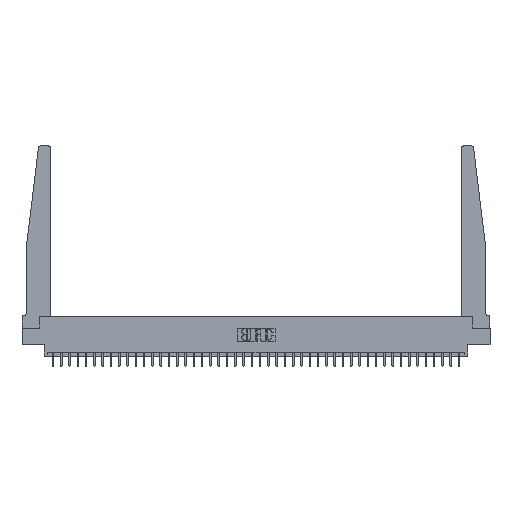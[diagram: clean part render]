
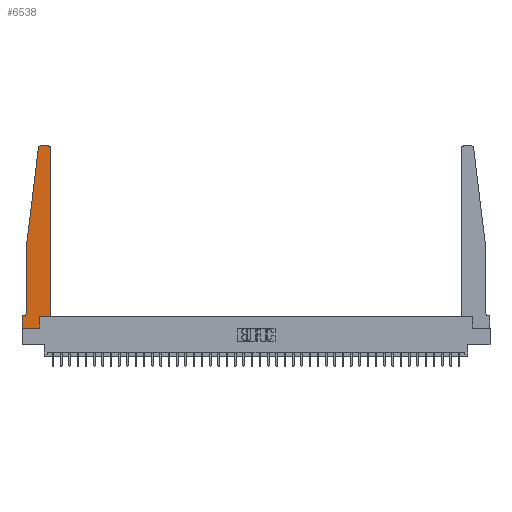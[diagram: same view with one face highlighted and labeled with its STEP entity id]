
A CAD part, top view. The second image highlights one B-rep face of the part: STEP entity #6538.
In plain terms, the highlighted planar face has unit normal (0, 0, 1).
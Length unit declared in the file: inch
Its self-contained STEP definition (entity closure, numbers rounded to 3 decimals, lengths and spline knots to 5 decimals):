
#1526 = CARTESIAN_POINT ( 'NONE',  ( 0.395, 2.72, 0.37 ) ) ;
#1542 = DIRECTION ( 'NONE',  ( 0., 0., -1. ) ) ;
#1617 = LINE ( 'NONE', #13007, #29551 ) ;
#2048 = ORIENTED_EDGE ( 'NONE', *, *, #34001, .T. ) ;
#3100 = EDGE_LOOP ( 'NONE', ( #33316, #14852, #31271, #36779, #28661, #2048, #5179, #14678, #21948, #8942, #9484, #10486 ) ) ;
#3137 = CARTESIAN_POINT ( 'NONE',  ( 0.2605, 0.18, 0.37 ) ) ;
#3719 = VECTOR ( 'NONE', #31763, 39.37008 ) ;
#3794 = VERTEX_POINT ( 'NONE', #31771 ) ;
#3957 = CARTESIAN_POINT ( 'NONE',  ( 0.27653, 2.75, 0.37 ) ) ;
#4169 = EDGE_CURVE ( 'NONE', #3794, #10725, #15048, .T. ) ;
#4283 = PLANE ( 'NONE',  #24182 ) ;
#4781 = DIRECTION ( 'NONE',  ( -1., 0., 0. ) ) ;
#5073 = VECTOR ( 'NONE', #5167, 39.37008 ) ;
#5167 = DIRECTION ( 'NONE',  ( 0., -1., 0. ) ) ;
#5179 = ORIENTED_EDGE ( 'NONE', *, *, #28534, .T. ) ;
#5540 = LINE ( 'NONE', #5727, #5073 ) ;
#5547 = VERTEX_POINT ( 'NONE', #3137 ) ;
#5727 = CARTESIAN_POINT ( 'NONE',  ( 0., 0., 0.37 ) ) ;
#5973 = VECTOR ( 'NONE', #20442, 39.37008 ) ;
#6538 = ADVANCED_FACE ( 'NONE', ( #36244 ), #4283, .T. ) ;
#6959 = DIRECTION ( 'NONE',  ( 0., 0., 1. ) ) ;
#6969 = DIRECTION ( 'NONE',  ( -1., 0., 0. ) ) ;
#7239 = DIRECTION ( 'NONE',  ( 1., 0., 0. ) ) ;
#7803 = EDGE_CURVE ( 'NONE', #36396, #22597, #21857, .T. ) ;
#8594 = LINE ( 'NONE', #34764, #9743 ) ;
#8942 = ORIENTED_EDGE ( 'NONE', *, *, #20430, .T. ) ;
#9484 = ORIENTED_EDGE ( 'NONE', *, *, #28379, .T. ) ;
#9743 = VECTOR ( 'NONE', #19972, 39.37008 ) ;
#9777 = CARTESIAN_POINT ( 'NONE',  ( 0.015, 0.2375, 0.37 ) ) ;
#9939 = DIRECTION ( 'NONE',  ( 0., 0., 1. ) ) ;
#10486 = ORIENTED_EDGE ( 'NONE', *, *, #7803, .T. ) ;
#10614 = DIRECTION ( 'NONE',  ( 0., 0., 1. ) ) ;
#10725 = VERTEX_POINT ( 'NONE', #16012 ) ;
#12377 = DIRECTION ( 'NONE',  ( 1., 0., 0. ) ) ;
#13007 = CARTESIAN_POINT ( 'NONE',  ( 0.425, 0.18, 0.37 ) ) ;
#13111 = DIRECTION ( 'NONE',  ( -1., 0., 0. ) ) ;
#13116 = CARTESIAN_POINT ( 'NONE',  ( 0.425, 0.18, 0.37 ) ) ;
#14678 = ORIENTED_EDGE ( 'NONE', *, *, #4169, .T. ) ;
#14852 = ORIENTED_EDGE ( 'NONE', *, *, #18160, .T. ) ;
#15007 = EDGE_CURVE ( 'NONE', #22597, #32096, #24589, .T. ) ;
#15048 = LINE ( 'NONE', #17679, #24041 ) ;
#15821 = CARTESIAN_POINT ( 'NONE',  ( 0.425, 2.72, 0.37 ) ) ;
#16012 = CARTESIAN_POINT ( 'NONE',  ( 0.2605, 0., 0.37 ) ) ;
#16172 = DIRECTION ( 'NONE',  ( 0., 1., 0. ) ) ;
#16971 = CARTESIAN_POINT ( 'NONE',  ( 0.2605, 0.18, 0.37 ) ) ;
#17413 = AXIS2_PLACEMENT_3D ( 'NONE', #29955, #6959, #23785 ) ;
#17631 = LINE ( 'NONE', #29066, #5973 ) ;
#17679 = CARTESIAN_POINT ( 'NONE',  ( 0., 0., 0.37 ) ) ;
#18160 = EDGE_CURVE ( 'NONE', #32096, #25208, #35925, .T. ) ;
#18832 = DIRECTION ( 'NONE',  ( 1., 0., 0. ) ) ;
#18935 = EDGE_CURVE ( 'NONE', #10725, #5547, #22770, .T. ) ;
#19972 = DIRECTION ( 'NONE',  ( -0.122, -0.992, 0. ) ) ;
#20430 = EDGE_CURVE ( 'NONE', #5547, #30534, #32678, .T. ) ;
#20442 = DIRECTION ( 'NONE',  ( 0., -1., 0. ) ) ;
#20759 = EDGE_CURVE ( 'NONE', #30481, #30093, #17631, .T. ) ;
#20985 = CARTESIAN_POINT ( 'NONE',  ( 0.065, 0.1875, 0.37 ) ) ;
#21250 = CARTESIAN_POINT ( 'NONE',  ( 0.425, 0.18, 0.37 ) ) ;
#21857 = CIRCLE ( 'NONE', #28442, 0.03 ) ;
#21948 = ORIENTED_EDGE ( 'NONE', *, *, #18935, .T. ) ;
#22597 = VERTEX_POINT ( 'NONE', #34638 ) ;
#22770 = LINE ( 'NONE', #16971, #3719 ) ;
#23251 = VECTOR ( 'NONE', #7239, 39.37008 ) ;
#23785 = DIRECTION ( 'NONE',  ( 1., 0., 0. ) ) ;
#24041 = VECTOR ( 'NONE', #29107, 39.37008 ) ;
#24182 = AXIS2_PLACEMENT_3D ( 'NONE', #33073, #10614, #18832 ) ;
#24332 = VERTEX_POINT ( 'NONE', #31254 ) ;
#24532 = CARTESIAN_POINT ( 'NONE',  ( 0.065, 1.25, 0.37 ) ) ;
#24589 = LINE ( 'NONE', #27761, #36380 ) ;
#25208 = VERTEX_POINT ( 'NONE', #36423 ) ;
#27370 = CARTESIAN_POINT ( 'NONE',  ( 0.065, 0.2375, 0.37 ) ) ;
#27761 = CARTESIAN_POINT ( 'NONE',  ( 0.25, 2.75, 0.37 ) ) ;
#28379 = EDGE_CURVE ( 'NONE', #30534, #36396, #1617, .T. ) ;
#28442 = AXIS2_PLACEMENT_3D ( 'NONE', #1526, #9939, #12377 ) ;
#28534 = EDGE_CURVE ( 'NONE', #30292, #3794, #5540, .T. ) ;
#28661 = ORIENTED_EDGE ( 'NONE', *, *, #35354, .T. ) ;
#28807 = CIRCLE ( 'NONE', #33601, 0.05 ) ;
#29066 = CARTESIAN_POINT ( 'NONE',  ( 0.065, 1.25, 0.37 ) ) ;
#29107 = DIRECTION ( 'NONE',  ( 1., 0., 0. ) ) ;
#29551 = VECTOR ( 'NONE', #16172, 39.37008 ) ;
#29955 = CARTESIAN_POINT ( 'NONE',  ( 0.27653, 2.72, 0.37 ) ) ;
#30093 = VERTEX_POINT ( 'NONE', #27370 ) ;
#30292 = VERTEX_POINT ( 'NONE', #35048 ) ;
#30481 = VERTEX_POINT ( 'NONE', #24532 ) ;
#30534 = VERTEX_POINT ( 'NONE', #13116 ) ;
#30949 = VECTOR ( 'NONE', #6969, 39.37008 ) ;
#31254 = CARTESIAN_POINT ( 'NONE',  ( 0.015, 0.1875, 0.37 ) ) ;
#31271 = ORIENTED_EDGE ( 'NONE', *, *, #36230, .T. ) ;
#31763 = DIRECTION ( 'NONE',  ( 0., 1., 0. ) ) ;
#31771 = CARTESIAN_POINT ( 'NONE',  ( 0., 0., 0.37 ) ) ;
#32096 = VERTEX_POINT ( 'NONE', #3957 ) ;
#32587 = LINE ( 'NONE', #20985, #30949 ) ;
#32678 = LINE ( 'NONE', #21250, #23251 ) ;
#33073 = CARTESIAN_POINT ( 'NONE',  ( 0., 0.1875, 0.37 ) ) ;
#33316 = ORIENTED_EDGE ( 'NONE', *, *, #15007, .T. ) ;
#33601 = AXIS2_PLACEMENT_3D ( 'NONE', #9777, #1542, #13111 ) ;
#34001 = EDGE_CURVE ( 'NONE', #24332, #30292, #32587, .T. ) ;
#34638 = CARTESIAN_POINT ( 'NONE',  ( 0.395, 2.75, 0.37 ) ) ;
#34764 = CARTESIAN_POINT ( 'NONE',  ( 0.065, 1.25, 0.37 ) ) ;
#35048 = CARTESIAN_POINT ( 'NONE',  ( 0., 0.1875, 0.37 ) ) ;
#35354 = EDGE_CURVE ( 'NONE', #30093, #24332, #28807, .T. ) ;
#35925 = CIRCLE ( 'NONE', #17413, 0.03 ) ;
#36230 = EDGE_CURVE ( 'NONE', #25208, #30481, #8594, .T. ) ;
#36244 = FACE_OUTER_BOUND ( 'NONE', #3100, .T. ) ;
#36380 = VECTOR ( 'NONE', #4781, 39.37008 ) ;
#36396 = VERTEX_POINT ( 'NONE', #15821 ) ;
#36423 = CARTESIAN_POINT ( 'NONE',  ( 0.24675, 2.72367, 0.37 ) ) ;
#36779 = ORIENTED_EDGE ( 'NONE', *, *, #20759, .T. ) ;
